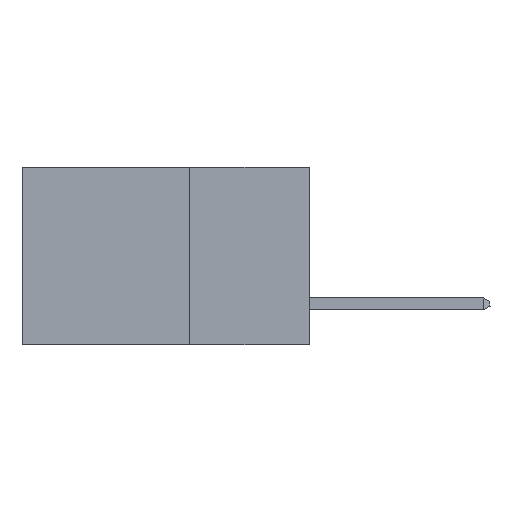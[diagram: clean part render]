
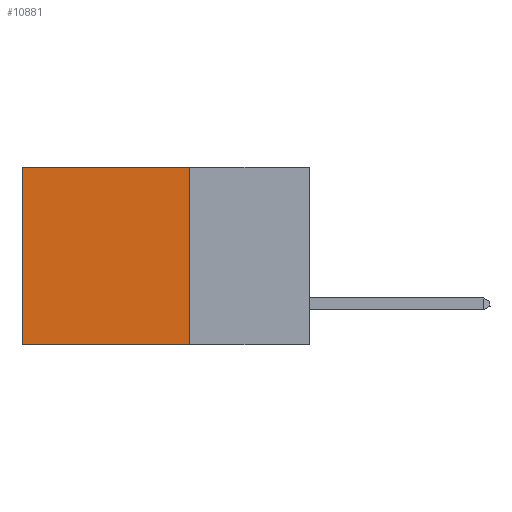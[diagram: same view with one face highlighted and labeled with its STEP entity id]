
A CAD part, left-side view. The second image highlights one B-rep face of the part: STEP entity #10881.
In plain terms, the highlighted planar face has unit normal (-1, 0, 0).
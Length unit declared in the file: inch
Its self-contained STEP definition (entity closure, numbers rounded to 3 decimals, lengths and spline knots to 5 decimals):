
#986 = CARTESIAN_POINT ( 'NONE',  ( 0.2875, 0.25, 0. ) ) ;
#1588 = CARTESIAN_POINT ( 'NONE',  ( 0.2875, 0.25, 0. ) ) ;
#1894 = DIRECTION ( 'NONE',  ( 0., 1., 0. ) ) ;
#2007 = VERTEX_POINT ( 'NONE', #1588 ) ;
#2832 = DIRECTION ( 'NONE',  ( 0., 1., 0. ) ) ;
#3415 = CARTESIAN_POINT ( 'NONE',  ( 0.2875, 0.25, 0. ) ) ;
#3982 = CARTESIAN_POINT ( 'NONE',  ( 0.2875, 0.6, -0.37 ) ) ;
#5165 = VERTEX_POINT ( 'NONE', #3982 ) ;
#5506 = ORIENTED_EDGE ( 'NONE', *, *, #16323, .T. ) ;
#5948 = DIRECTION ( 'NONE',  ( 0., 0., -1. ) ) ;
#6062 = PLANE ( 'NONE',  #6295 ) ;
#6165 = EDGE_LOOP ( 'NONE', ( #13797, #7917, #15450, #5506 ) ) ;
#6231 = VECTOR ( 'NONE', #5948, 39.37008 ) ;
#6295 = AXIS2_PLACEMENT_3D ( 'NONE', #3415, #14991, #7371 ) ;
#7196 = CARTESIAN_POINT ( 'NONE',  ( 0.2875, 0.6, 0. ) ) ;
#7371 = DIRECTION ( 'NONE',  ( 0., 0., -1. ) ) ;
#7917 = ORIENTED_EDGE ( 'NONE', *, *, #9500, .F. ) ;
#8354 = LINE ( 'NONE', #986, #11417 ) ;
#8874 = FACE_OUTER_BOUND ( 'NONE', #6165, .T. ) ;
#8999 = DIRECTION ( 'NONE',  ( 0., 0., -1. ) ) ;
#9500 = EDGE_CURVE ( 'NONE', #15859, #5165, #11363, .T. ) ;
#9790 = CARTESIAN_POINT ( 'NONE',  ( 0.2875, 0.25, -0.37 ) ) ;
#9981 = CARTESIAN_POINT ( 'NONE',  ( 0.2875, 0.6, 0. ) ) ;
#10708 = CARTESIAN_POINT ( 'NONE',  ( 0.2875, 0.25, 0. ) ) ;
#10823 = EDGE_CURVE ( 'NONE', #12716, #5165, #13464, .T. ) ;
#10881 = ADVANCED_FACE ( 'NONE', ( #8874 ), #6062, .F. ) ;
#11363 = LINE ( 'NONE', #9790, #14669 ) ;
#11417 = VECTOR ( 'NONE', #8999, 39.37008 ) ;
#12438 = VECTOR ( 'NONE', #2832, 39.37008 ) ;
#12716 = VERTEX_POINT ( 'NONE', #9981 ) ;
#13210 = LINE ( 'NONE', #10708, #12438 ) ;
#13430 = EDGE_CURVE ( 'NONE', #2007, #15859, #8354, .T. ) ;
#13464 = LINE ( 'NONE', #7196, #6231 ) ;
#13797 = ORIENTED_EDGE ( 'NONE', *, *, #10823, .T. ) ;
#14528 = CARTESIAN_POINT ( 'NONE',  ( 0.2875, 0.25, -0.37 ) ) ;
#14669 = VECTOR ( 'NONE', #1894, 39.37008 ) ;
#14991 = DIRECTION ( 'NONE',  ( 1., 0., 0. ) ) ;
#15450 = ORIENTED_EDGE ( 'NONE', *, *, #13430, .F. ) ;
#15859 = VERTEX_POINT ( 'NONE', #14528 ) ;
#16323 = EDGE_CURVE ( 'NONE', #2007, #12716, #13210, .T. ) ;
